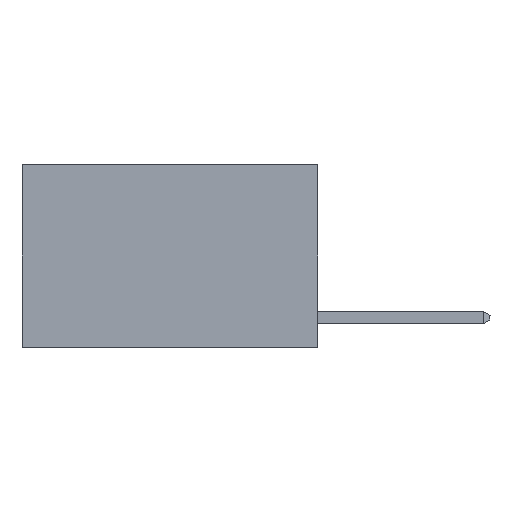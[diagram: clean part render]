
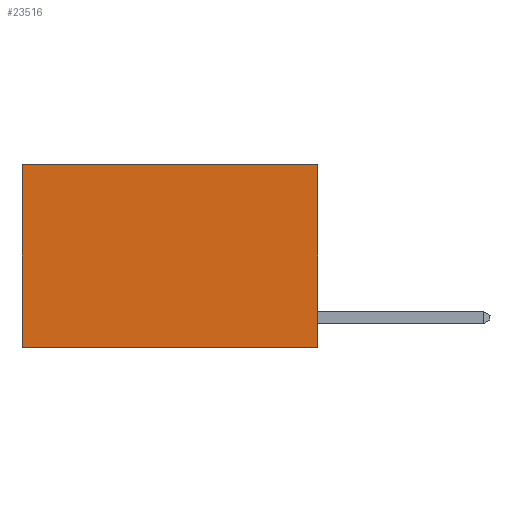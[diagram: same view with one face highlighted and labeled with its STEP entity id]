
A CAD part, left-side view. The second image highlights one B-rep face of the part: STEP entity #23516.
In plain terms, the highlighted planar face has unit normal (-1, 0, 0).
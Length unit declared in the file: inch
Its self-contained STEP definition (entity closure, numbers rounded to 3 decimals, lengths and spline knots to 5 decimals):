
#136 = PLANE ( 'NONE',  #15448 ) ;
#1190 = CARTESIAN_POINT ( 'NONE',  ( 0.2625, 0.6, 0. ) ) ;
#1529 = VECTOR ( 'NONE', #22203, 39.37008 ) ;
#2704 = VECTOR ( 'NONE', #4703, 39.37008 ) ;
#3345 = EDGE_CURVE ( 'NONE', #18737, #10014, #7248, .T. ) ;
#3350 = LINE ( 'NONE', #13448, #22656 ) ;
#4448 = LINE ( 'NONE', #21608, #16656 ) ;
#4703 = DIRECTION ( 'NONE',  ( 0., 1., 0. ) ) ;
#5466 = CARTESIAN_POINT ( 'NONE',  ( 0.2625, 0., -0.37 ) ) ;
#7248 = LINE ( 'NONE', #12207, #2704 ) ;
#8495 = EDGE_CURVE ( 'NONE', #24034, #10014, #4448, .T. ) ;
#9729 = ORIENTED_EDGE ( 'NONE', *, *, #8495, .T. ) ;
#10014 = VERTEX_POINT ( 'NONE', #23657 ) ;
#10409 = ORIENTED_EDGE ( 'NONE', *, *, #3345, .F. ) ;
#10863 = DIRECTION ( 'NONE',  ( 1., 0., 0. ) ) ;
#12207 = CARTESIAN_POINT ( 'NONE',  ( 0.2625, 0., -0.37 ) ) ;
#12265 = FACE_OUTER_BOUND ( 'NONE', #14825, .T. ) ;
#13386 = CARTESIAN_POINT ( 'NONE',  ( 0.2625, 0., 0. ) ) ;
#13448 = CARTESIAN_POINT ( 'NONE',  ( 0.2625, 0., 0. ) ) ;
#13499 = DIRECTION ( 'NONE',  ( 0., 0., -1. ) ) ;
#14252 = CARTESIAN_POINT ( 'NONE',  ( 0.2625, 0., 0. ) ) ;
#14825 = EDGE_LOOP ( 'NONE', ( #9729, #10409, #26279, #23528 ) ) ;
#15448 = AXIS2_PLACEMENT_3D ( 'NONE', #25405, #10863, #25308 ) ;
#15731 = LINE ( 'NONE', #14252, #1529 ) ;
#16575 = EDGE_CURVE ( 'NONE', #20929, #18737, #15731, .T. ) ;
#16656 = VECTOR ( 'NONE', #13499, 39.37008 ) ;
#18737 = VERTEX_POINT ( 'NONE', #5466 ) ;
#20929 = VERTEX_POINT ( 'NONE', #13386 ) ;
#21456 = EDGE_CURVE ( 'NONE', #20929, #24034, #3350, .T. ) ;
#21608 = CARTESIAN_POINT ( 'NONE',  ( 0.2625, 0.6, 0. ) ) ;
#21656 = DIRECTION ( 'NONE',  ( 0., 1., 0. ) ) ;
#22203 = DIRECTION ( 'NONE',  ( 0., 0., -1. ) ) ;
#22656 = VECTOR ( 'NONE', #21656, 39.37008 ) ;
#23516 = ADVANCED_FACE ( 'NONE', ( #12265 ), #136, .F. ) ;
#23528 = ORIENTED_EDGE ( 'NONE', *, *, #21456, .T. ) ;
#23657 = CARTESIAN_POINT ( 'NONE',  ( 0.2625, 0.6, -0.37 ) ) ;
#24034 = VERTEX_POINT ( 'NONE', #1190 ) ;
#25308 = DIRECTION ( 'NONE',  ( 0., 0., -1. ) ) ;
#25405 = CARTESIAN_POINT ( 'NONE',  ( 0.2625, 0., 0. ) ) ;
#26279 = ORIENTED_EDGE ( 'NONE', *, *, #16575, .F. ) ;
